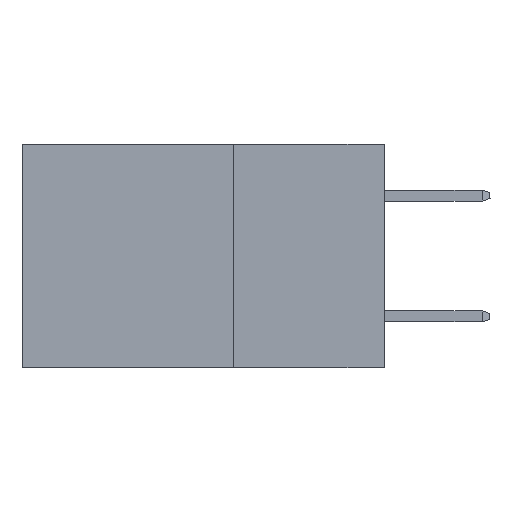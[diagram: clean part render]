
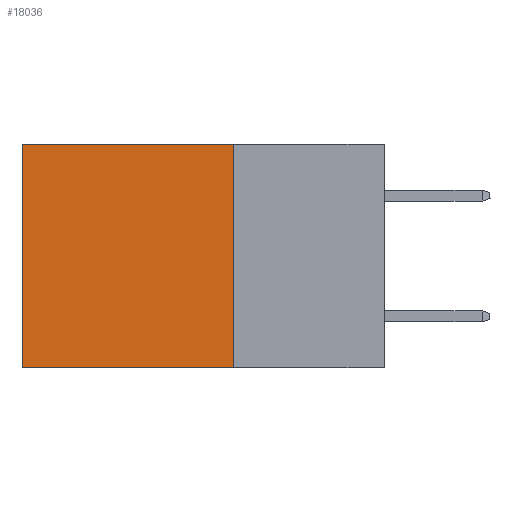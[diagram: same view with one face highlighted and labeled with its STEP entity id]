
A CAD part, left-side view. The second image highlights one B-rep face of the part: STEP entity #18036.
In plain terms, the highlighted planar face has unit normal (-1, 0, 0).
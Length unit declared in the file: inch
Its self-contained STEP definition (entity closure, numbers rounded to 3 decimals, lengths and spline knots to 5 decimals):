
#269 = VERTEX_POINT ( 'NONE', #8324 ) ;
#443 = ORIENTED_EDGE ( 'NONE', *, *, #12808, .F. ) ;
#1149 = LINE ( 'NONE', #18949, #20359 ) ;
#1213 = EDGE_LOOP ( 'NONE', ( #2850, #3576, #443, #11730 ) ) ;
#2441 = CARTESIAN_POINT ( 'NONE',  ( 0.298, 0.25, -0.37 ) ) ;
#2850 = ORIENTED_EDGE ( 'NONE', *, *, #10457, .T. ) ;
#3576 = ORIENTED_EDGE ( 'NONE', *, *, #22936, .F. ) ;
#3867 = VERTEX_POINT ( 'NONE', #20973 ) ;
#4228 = PLANE ( 'NONE',  #9465 ) ;
#5762 = CARTESIAN_POINT ( 'NONE',  ( 0.298, 0.25, -0.37 ) ) ;
#6147 = CARTESIAN_POINT ( 'NONE',  ( 0.298, 0.25, 0. ) ) ;
#6221 = DIRECTION ( 'NONE',  ( 0., 0., -1. ) ) ;
#7776 = FACE_OUTER_BOUND ( 'NONE', #1213, .T. ) ;
#8103 = DIRECTION ( 'NONE',  ( 0., 0., -1. ) ) ;
#8324 = CARTESIAN_POINT ( 'NONE',  ( 0.298, 0.25, 0. ) ) ;
#8984 = VECTOR ( 'NONE', #8103, 39.37008 ) ;
#9465 = AXIS2_PLACEMENT_3D ( 'NONE', #23285, #17669, #6221 ) ;
#9505 = DIRECTION ( 'NONE',  ( 0., 1., 0. ) ) ;
#10279 = VERTEX_POINT ( 'NONE', #5762 ) ;
#10457 = EDGE_CURVE ( 'NONE', #3867, #19178, #22164, .T. ) ;
#11730 = ORIENTED_EDGE ( 'NONE', *, *, #15179, .T. ) ;
#11758 = VECTOR ( 'NONE', #19681, 39.37008 ) ;
#12808 = EDGE_CURVE ( 'NONE', #269, #10279, #18509, .T. ) ;
#15179 = EDGE_CURVE ( 'NONE', #269, #3867, #1149, .T. ) ;
#15801 = DIRECTION ( 'NONE',  ( 0., 0., -1. ) ) ;
#16819 = LINE ( 'NONE', #2441, #11758 ) ;
#17430 = CARTESIAN_POINT ( 'NONE',  ( 0.298, 0.6, -0.37 ) ) ;
#17669 = DIRECTION ( 'NONE',  ( 1., 0., 0. ) ) ;
#17715 = CARTESIAN_POINT ( 'NONE',  ( 0.298, 0.6, 0. ) ) ;
#18036 = ADVANCED_FACE ( 'NONE', ( #7776 ), #4228, .F. ) ;
#18509 = LINE ( 'NONE', #6147, #8984 ) ;
#18949 = CARTESIAN_POINT ( 'NONE',  ( 0.298, 0.25, 0. ) ) ;
#19178 = VERTEX_POINT ( 'NONE', #17430 ) ;
#19681 = DIRECTION ( 'NONE',  ( 0., 1., 0. ) ) ;
#20359 = VECTOR ( 'NONE', #9505, 39.37008 ) ;
#20973 = CARTESIAN_POINT ( 'NONE',  ( 0.298, 0.6, 0. ) ) ;
#21568 = VECTOR ( 'NONE', #15801, 39.37008 ) ;
#22164 = LINE ( 'NONE', #17715, #21568 ) ;
#22936 = EDGE_CURVE ( 'NONE', #10279, #19178, #16819, .T. ) ;
#23285 = CARTESIAN_POINT ( 'NONE',  ( 0.298, 0.25, 0. ) ) ;
